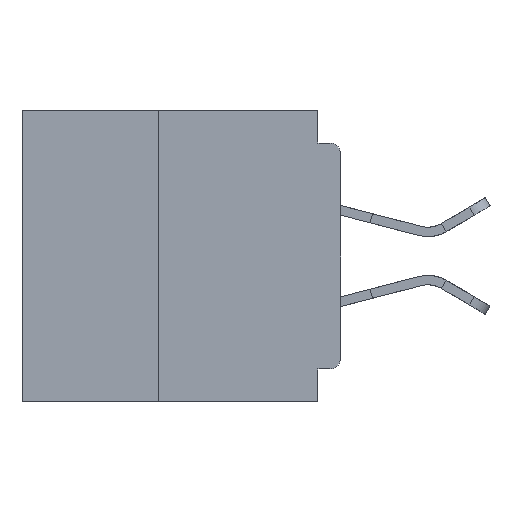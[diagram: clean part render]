
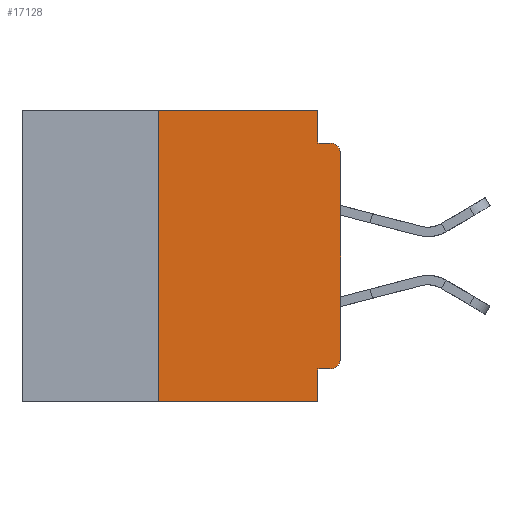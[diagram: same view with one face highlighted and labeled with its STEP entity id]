
A CAD part, left-side view. The second image highlights one B-rep face of the part: STEP entity #17128.
In plain terms, the highlighted planar face has unit normal (-1, 0, 0).
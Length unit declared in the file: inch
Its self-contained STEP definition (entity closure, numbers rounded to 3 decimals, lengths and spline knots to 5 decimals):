
#705 = LINE ( 'NONE', #7799, #42449 ) ;
#994 = DIRECTION ( 'NONE',  ( 0., 0., 1. ) ) ;
#1585 = CARTESIAN_POINT ( 'NONE',  ( 0., 0.031, -0.355 ) ) ;
#1894 = DIRECTION ( 'NONE',  ( 0., 1., 0. ) ) ;
#2743 = LINE ( 'NONE', #42366, #28872 ) ;
#3333 = ORIENTED_EDGE ( 'NONE', *, *, #15610, .F. ) ;
#4185 = CARTESIAN_POINT ( 'NONE',  ( 0., 0.015, -0.045 ) ) ;
#4257 = AXIS2_PLACEMENT_3D ( 'NONE', #26739, #6369, #30102 ) ;
#4558 = EDGE_LOOP ( 'NONE', ( #41096, #15360, #3333, #10673, #29155, #9878, #29747, #22841, #10387, #42601 ) ) ;
#4838 = EDGE_CURVE ( 'NONE', #8311, #33005, #29263, .T. ) ;
#6041 = DIRECTION ( 'NONE',  ( 0., 0., -1. ) ) ;
#6179 = CIRCLE ( 'NONE', #4257, 0.015 ) ;
#6369 = DIRECTION ( 'NONE',  ( -1., 0., 0. ) ) ;
#6635 = VECTOR ( 'NONE', #6749, 39.37008 ) ;
#6749 = DIRECTION ( 'NONE',  ( 0., 0., -1. ) ) ;
#7188 = DIRECTION ( 'NONE',  ( -1., 0., 0. ) ) ;
#7423 = LINE ( 'NONE', #13904, #23390 ) ;
#7746 = DIRECTION ( 'NONE',  ( 0., 0., -1. ) ) ;
#7799 = CARTESIAN_POINT ( 'NONE',  ( 0., 0.437, -0.4 ) ) ;
#8230 = LINE ( 'NONE', #32565, #42910 ) ;
#8311 = VERTEX_POINT ( 'NONE', #25509 ) ;
#9878 = ORIENTED_EDGE ( 'NONE', *, *, #25983, .F. ) ;
#10387 = ORIENTED_EDGE ( 'NONE', *, *, #30397, .F. ) ;
#10673 = ORIENTED_EDGE ( 'NONE', *, *, #43166, .F. ) ;
#11381 = VERTEX_POINT ( 'NONE', #31554 ) ;
#12026 = VERTEX_POINT ( 'NONE', #31657 ) ;
#12093 = VECTOR ( 'NONE', #6041, 39.37008 ) ;
#13355 = EDGE_CURVE ( 'NONE', #21969, #28456, #36858, .T. ) ;
#13904 = CARTESIAN_POINT ( 'NONE',  ( 0., 0.25, -0.4 ) ) ;
#14444 = CARTESIAN_POINT ( 'NONE',  ( 0., 0.437, 0. ) ) ;
#14820 = CARTESIAN_POINT ( 'NONE',  ( 0., 0., 0. ) ) ;
#15360 = ORIENTED_EDGE ( 'NONE', *, *, #41959, .T. ) ;
#15381 = VECTOR ( 'NONE', #27090, 39.37008 ) ;
#15610 = EDGE_CURVE ( 'NONE', #11381, #40123, #8230, .T. ) ;
#16955 = CARTESIAN_POINT ( 'NONE',  ( 0., 0.031, -0.4 ) ) ;
#17128 = ADVANCED_FACE ( 'NONE', ( #42143 ), #17697, .F. ) ;
#17697 = PLANE ( 'NONE',  #23657 ) ;
#18318 = AXIS2_PLACEMENT_3D ( 'NONE', #27514, #7188, #30874 ) ;
#20566 = CARTESIAN_POINT ( 'NONE',  ( 0., 0.25, 0. ) ) ;
#20574 = CARTESIAN_POINT ( 'NONE',  ( 0., 0.437, 0. ) ) ;
#21969 = VERTEX_POINT ( 'NONE', #1585 ) ;
#22841 = ORIENTED_EDGE ( 'NONE', *, *, #13355, .F. ) ;
#23390 = VECTOR ( 'NONE', #37430, 39.37008 ) ;
#23657 = AXIS2_PLACEMENT_3D ( 'NONE', #14444, #28053, #7746 ) ;
#23734 = CARTESIAN_POINT ( 'NONE',  ( 0., 0.031, 0. ) ) ;
#25479 = LINE ( 'NONE', #20574, #15381 ) ;
#25509 = CARTESIAN_POINT ( 'NONE',  ( 0., 0.015, -0.355 ) ) ;
#25951 = EDGE_CURVE ( 'NONE', #41447, #12026, #25479, .T. ) ;
#25983 = EDGE_CURVE ( 'NONE', #36649, #41447, #7423, .T. ) ;
#26418 = CARTESIAN_POINT ( 'NONE',  ( 0., 0.031, -0.4 ) ) ;
#26739 = CARTESIAN_POINT ( 'NONE',  ( 0., 0.015, -0.06 ) ) ;
#26824 = CARTESIAN_POINT ( 'NONE',  ( 0., 0.25, -0.4 ) ) ;
#27018 = CARTESIAN_POINT ( 'NONE',  ( 0., 0., -0.34 ) ) ;
#27090 = DIRECTION ( 'NONE',  ( 0., -1., 0. ) ) ;
#27514 = CARTESIAN_POINT ( 'NONE',  ( 0., 0.015, -0.34 ) ) ;
#27997 = EDGE_CURVE ( 'NONE', #36649, #28456, #705, .T. ) ;
#28053 = DIRECTION ( 'NONE',  ( 1., 0., 0. ) ) ;
#28456 = VERTEX_POINT ( 'NONE', #16955 ) ;
#28872 = VECTOR ( 'NONE', #1894, 39.37008 ) ;
#29155 = ORIENTED_EDGE ( 'NONE', *, *, #25951, .F. ) ;
#29263 = CIRCLE ( 'NONE', #18318, 0.015 ) ;
#29300 = EDGE_CURVE ( 'NONE', #33005, #31296, #36273, .T. ) ;
#29315 = DIRECTION ( 'NONE',  ( 0., -1., 0. ) ) ;
#29747 = ORIENTED_EDGE ( 'NONE', *, *, #27997, .T. ) ;
#30102 = DIRECTION ( 'NONE',  ( 0., 0., -1. ) ) ;
#30397 = EDGE_CURVE ( 'NONE', #8311, #21969, #2743, .T. ) ;
#30874 = DIRECTION ( 'NONE',  ( 0., 0., -1. ) ) ;
#31296 = VERTEX_POINT ( 'NONE', #37416 ) ;
#31476 = DIRECTION ( 'NONE',  ( 0., -1., 0. ) ) ;
#31554 = CARTESIAN_POINT ( 'NONE',  ( 0., 0.031, -0.045 ) ) ;
#31657 = CARTESIAN_POINT ( 'NONE',  ( 0., 0.031, 0. ) ) ;
#32565 = CARTESIAN_POINT ( 'NONE',  ( 0., 0., -0.045 ) ) ;
#33005 = VERTEX_POINT ( 'NONE', #27018 ) ;
#33661 = LINE ( 'NONE', #23734, #6635 ) ;
#35239 = VECTOR ( 'NONE', #994, 39.37008 ) ;
#36273 = LINE ( 'NONE', #14820, #35239 ) ;
#36649 = VERTEX_POINT ( 'NONE', #26824 ) ;
#36858 = LINE ( 'NONE', #26418, #12093 ) ;
#37416 = CARTESIAN_POINT ( 'NONE',  ( 0., 0., -0.06 ) ) ;
#37430 = DIRECTION ( 'NONE',  ( 0., 0., 1. ) ) ;
#40123 = VERTEX_POINT ( 'NONE', #4185 ) ;
#41096 = ORIENTED_EDGE ( 'NONE', *, *, #29300, .T. ) ;
#41447 = VERTEX_POINT ( 'NONE', #20566 ) ;
#41959 = EDGE_CURVE ( 'NONE', #31296, #40123, #6179, .T. ) ;
#42143 = FACE_OUTER_BOUND ( 'NONE', #4558, .T. ) ;
#42366 = CARTESIAN_POINT ( 'NONE',  ( 0., 0., -0.355 ) ) ;
#42449 = VECTOR ( 'NONE', #31476, 39.37008 ) ;
#42601 = ORIENTED_EDGE ( 'NONE', *, *, #4838, .T. ) ;
#42910 = VECTOR ( 'NONE', #29315, 39.37008 ) ;
#43166 = EDGE_CURVE ( 'NONE', #12026, #11381, #33661, .T. ) ;
